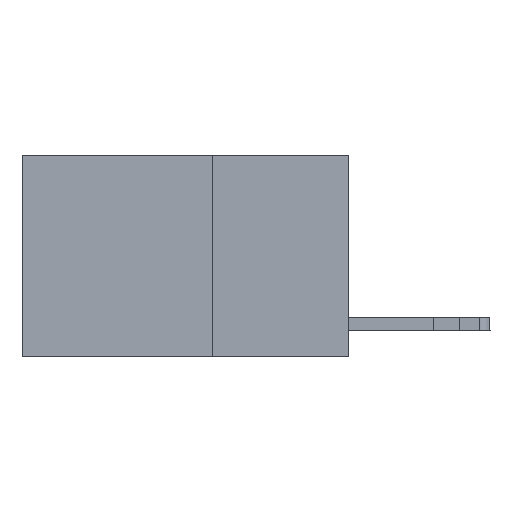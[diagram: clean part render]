
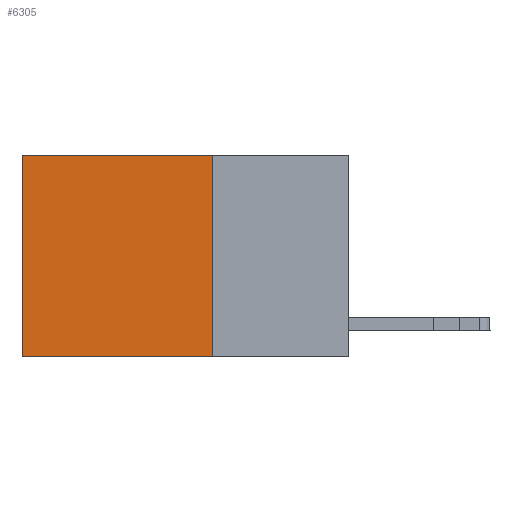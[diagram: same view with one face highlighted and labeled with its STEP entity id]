
A CAD part, left-side view. The second image highlights one B-rep face of the part: STEP entity #6305.
In plain terms, the highlighted planar face has unit normal (-1, 0, 0).
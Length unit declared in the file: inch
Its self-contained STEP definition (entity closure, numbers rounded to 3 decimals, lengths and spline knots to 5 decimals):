
#363 = EDGE_CURVE ( 'NONE', #18399, #14300, #14418, .T. ) ;
#1193 = LINE ( 'NONE', #12097, #7959 ) ;
#1481 = LINE ( 'NONE', #3022, #13445 ) ;
#1552 = ORIENTED_EDGE ( 'NONE', *, *, #363, .T. ) ;
#1561 = CARTESIAN_POINT ( 'NONE',  ( 0.2625, 0.25, 0. ) ) ;
#1731 = DIRECTION ( 'NONE',  ( 0., 0., -1. ) ) ;
#2499 = DIRECTION ( 'NONE',  ( 0., 0., -1. ) ) ;
#3022 = CARTESIAN_POINT ( 'NONE',  ( 0.2625, 0.25, -0.37 ) ) ;
#3032 = VERTEX_POINT ( 'NONE', #19612 ) ;
#4511 = CARTESIAN_POINT ( 'NONE',  ( 0.2625, 0.25, 0. ) ) ;
#4707 = LINE ( 'NONE', #24013, #7324 ) ;
#5160 = DIRECTION ( 'NONE',  ( 1., 0., 0. ) ) ;
#6305 = ADVANCED_FACE ( 'NONE', ( #22085 ), #13268, .F. ) ;
#6849 = EDGE_CURVE ( 'NONE', #14300, #3032, #4707, .T. ) ;
#7324 = VECTOR ( 'NONE', #19807, 39.37008 ) ;
#7800 = ORIENTED_EDGE ( 'NONE', *, *, #6849, .T. ) ;
#7959 = VECTOR ( 'NONE', #1731, 39.37008 ) ;
#8060 = VERTEX_POINT ( 'NONE', #26001 ) ;
#8179 = CARTESIAN_POINT ( 'NONE',  ( 0.2625, 0.6, 0. ) ) ;
#12097 = CARTESIAN_POINT ( 'NONE',  ( 0.2625, 0.25, 0. ) ) ;
#13108 = EDGE_CURVE ( 'NONE', #18399, #8060, #1193, .T. ) ;
#13268 = PLANE ( 'NONE',  #26947 ) ;
#13272 = ORIENTED_EDGE ( 'NONE', *, *, #13108, .F. ) ;
#13445 = VECTOR ( 'NONE', #13660, 39.37008 ) ;
#13660 = DIRECTION ( 'NONE',  ( 0., 1., 0. ) ) ;
#14300 = VERTEX_POINT ( 'NONE', #8179 ) ;
#14418 = LINE ( 'NONE', #1561, #27653 ) ;
#16275 = EDGE_CURVE ( 'NONE', #8060, #3032, #1481, .T. ) ;
#18399 = VERTEX_POINT ( 'NONE', #4511 ) ;
#18622 = DIRECTION ( 'NONE',  ( 0., 1., 0. ) ) ;
#19612 = CARTESIAN_POINT ( 'NONE',  ( 0.2625, 0.6, -0.37 ) ) ;
#19807 = DIRECTION ( 'NONE',  ( 0., 0., -1. ) ) ;
#22085 = FACE_OUTER_BOUND ( 'NONE', #26526, .T. ) ;
#22214 = CARTESIAN_POINT ( 'NONE',  ( 0.2625, 0.25, 0. ) ) ;
#23642 = ORIENTED_EDGE ( 'NONE', *, *, #16275, .F. ) ;
#24013 = CARTESIAN_POINT ( 'NONE',  ( 0.2625, 0.6, 0. ) ) ;
#26001 = CARTESIAN_POINT ( 'NONE',  ( 0.2625, 0.25, -0.37 ) ) ;
#26526 = EDGE_LOOP ( 'NONE', ( #7800, #23642, #13272, #1552 ) ) ;
#26947 = AXIS2_PLACEMENT_3D ( 'NONE', #22214, #5160, #2499 ) ;
#27653 = VECTOR ( 'NONE', #18622, 39.37008 ) ;
